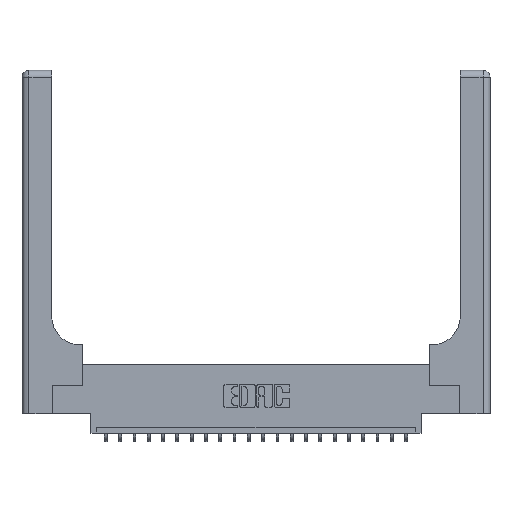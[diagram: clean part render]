
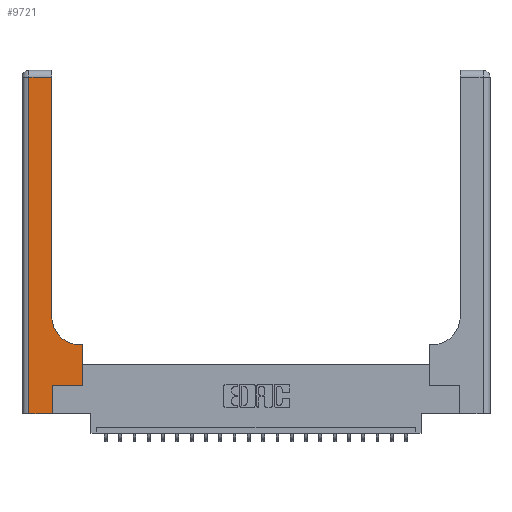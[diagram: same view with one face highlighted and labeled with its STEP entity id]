
A CAD part, top view. The second image highlights one B-rep face of the part: STEP entity #9721.
In plain terms, the highlighted planar face has unit normal (0, 0, 1).
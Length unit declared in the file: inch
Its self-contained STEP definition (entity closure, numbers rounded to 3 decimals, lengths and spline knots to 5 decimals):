
#112 = CARTESIAN_POINT ( 'NONE',  ( 0.26, 0.85, 0.37 ) ) ;
#235 = ORIENTED_EDGE ( 'NONE', *, *, #10146, .T. ) ;
#906 = DIRECTION ( 'NONE',  ( 0., -1., 0. ) ) ;
#1063 = ORIENTED_EDGE ( 'NONE', *, *, #17139, .T. ) ;
#1160 = VERTEX_POINT ( 'NONE', #5119 ) ;
#1161 = FACE_OUTER_BOUND ( 'NONE', #1976, .T. ) ;
#1162 = DIRECTION ( 'NONE',  ( 0., 0., -1. ) ) ;
#1529 = LINE ( 'NONE', #20406, #5972 ) ;
#1976 = EDGE_LOOP ( 'NONE', ( #15490, #3197, #235, #1063, #12956, #17409, #16443, #17514, #17285 ) ) ;
#1989 = DIRECTION ( 'NONE',  ( 1., 0., 0. ) ) ;
#2248 = DIRECTION ( 'NONE',  ( 0., 1., 0. ) ) ;
#2731 = DIRECTION ( 'NONE',  ( 0., 0., -1. ) ) ;
#2846 = VERTEX_POINT ( 'NONE', #6598 ) ;
#3197 = ORIENTED_EDGE ( 'NONE', *, *, #6255, .T. ) ;
#3683 = VERTEX_POINT ( 'NONE', #14350 ) ;
#3777 = AXIS2_PLACEMENT_3D ( 'NONE', #12794, #2731, #14482 ) ;
#4137 = EDGE_CURVE ( 'NONE', #20984, #18378, #16483, .T. ) ;
#4300 = LINE ( 'NONE', #13992, #12717 ) ;
#5119 = CARTESIAN_POINT ( 'NONE',  ( 0.265, 0., 0.37 ) ) ;
#5766 = DIRECTION ( 'NONE',  ( -1., 0., 0. ) ) ;
#5972 = VECTOR ( 'NONE', #1989, 39.37008 ) ;
#6255 = EDGE_CURVE ( 'NONE', #3683, #18722, #9473, .T. ) ;
#6491 = VERTEX_POINT ( 'NONE', #19891 ) ;
#6598 = CARTESIAN_POINT ( 'NONE',  ( 0.06, 0., 0.37 ) ) ;
#7945 = EDGE_CURVE ( 'NONE', #6491, #11851, #12534, .T. ) ;
#7980 = CARTESIAN_POINT ( 'NONE',  ( 0.265, 0.25, 0.37 ) ) ;
#8054 = VECTOR ( 'NONE', #10459, 39.37008 ) ;
#8593 = LINE ( 'NONE', #15505, #8054 ) ;
#9389 = CARTESIAN_POINT ( 'NONE',  ( 0.26, 3., 0.37 ) ) ;
#9473 = LINE ( 'NONE', #17550, #13929 ) ;
#9721 = ADVANCED_FACE ( 'NONE', ( #1161 ), #21280, .F. ) ;
#10034 = EDGE_CURVE ( 'NONE', #1160, #11745, #4300, .T. ) ;
#10146 = EDGE_CURVE ( 'NONE', #18722, #2846, #19544, .T. ) ;
#10301 = EDGE_CURVE ( 'NONE', #11745, #6491, #16922, .T. ) ;
#10459 = DIRECTION ( 'NONE',  ( -1., 0., 0. ) ) ;
#10983 = CARTESIAN_POINT ( 'NONE',  ( 0.06, 3., 0.37 ) ) ;
#11128 = VECTOR ( 'NONE', #906, 39.37008 ) ;
#11230 = CARTESIAN_POINT ( 'NONE',  ( 0., 3., 0.37 ) ) ;
#11745 = VERTEX_POINT ( 'NONE', #11876 ) ;
#11851 = VERTEX_POINT ( 'NONE', #15525 ) ;
#11876 = CARTESIAN_POINT ( 'NONE',  ( 0.265, 0.25, 0.37 ) ) ;
#12352 = CARTESIAN_POINT ( 'NONE',  ( 0.528, 0.25, 0.37 ) ) ;
#12534 = LINE ( 'NONE', #12352, #20937 ) ;
#12717 = VECTOR ( 'NONE', #2248, 39.37008 ) ;
#12794 = CARTESIAN_POINT ( 'NONE',  ( 0.51, 0.85, 0.37 ) ) ;
#12921 = DIRECTION ( 'NONE',  ( -1., 0., 0. ) ) ;
#12956 = ORIENTED_EDGE ( 'NONE', *, *, #10034, .T. ) ;
#13929 = VECTOR ( 'NONE', #5766, 39.37008 ) ;
#13992 = CARTESIAN_POINT ( 'NONE',  ( 0.265, 0., 0.37 ) ) ;
#14052 = DIRECTION ( 'NONE',  ( 0., 1., 0. ) ) ;
#14350 = CARTESIAN_POINT ( 'NONE',  ( 0.26, 2.94, 0.37 ) ) ;
#14482 = DIRECTION ( 'NONE',  ( 1., 0., 0. ) ) ;
#14678 = DIRECTION ( 'NONE',  ( 1., 0., 0. ) ) ;
#15490 = ORIENTED_EDGE ( 'NONE', *, *, #17411, .T. ) ;
#15505 = CARTESIAN_POINT ( 'NONE',  ( 0.26, 0.6, 0.37 ) ) ;
#15525 = CARTESIAN_POINT ( 'NONE',  ( 0.528, 0.6, 0.37 ) ) ;
#16443 = ORIENTED_EDGE ( 'NONE', *, *, #7945, .T. ) ;
#16483 = CIRCLE ( 'NONE', #3777, 0.25 ) ;
#16922 = LINE ( 'NONE', #7980, #21364 ) ;
#17139 = EDGE_CURVE ( 'NONE', #2846, #1160, #1529, .T. ) ;
#17285 = ORIENTED_EDGE ( 'NONE', *, *, #4137, .T. ) ;
#17409 = ORIENTED_EDGE ( 'NONE', *, *, #10301, .T. ) ;
#17411 = EDGE_CURVE ( 'NONE', #18378, #3683, #19124, .T. ) ;
#17514 = ORIENTED_EDGE ( 'NONE', *, *, #18509, .T. ) ;
#17550 = CARTESIAN_POINT ( 'NONE',  ( 0., 2.94, 0.37 ) ) ;
#17681 = AXIS2_PLACEMENT_3D ( 'NONE', #11230, #1162, #12921 ) ;
#18071 = CARTESIAN_POINT ( 'NONE',  ( 0.06, 2.94, 0.37 ) ) ;
#18378 = VERTEX_POINT ( 'NONE', #112 ) ;
#18509 = EDGE_CURVE ( 'NONE', #11851, #20984, #8593, .T. ) ;
#18722 = VERTEX_POINT ( 'NONE', #18071 ) ;
#19124 = LINE ( 'NONE', #9389, #19647 ) ;
#19544 = LINE ( 'NONE', #10983, #11128 ) ;
#19647 = VECTOR ( 'NONE', #21126, 39.37008 ) ;
#19891 = CARTESIAN_POINT ( 'NONE',  ( 0.528, 0.25, 0.37 ) ) ;
#20406 = CARTESIAN_POINT ( 'NONE',  ( 0., 0., 0.37 ) ) ;
#20937 = VECTOR ( 'NONE', #14052, 39.37008 ) ;
#20984 = VERTEX_POINT ( 'NONE', #21584 ) ;
#21126 = DIRECTION ( 'NONE',  ( 0., 1., 0. ) ) ;
#21280 = PLANE ( 'NONE',  #17681 ) ;
#21364 = VECTOR ( 'NONE', #14678, 39.37008 ) ;
#21584 = CARTESIAN_POINT ( 'NONE',  ( 0.51, 0.6, 0.37 ) ) ;
